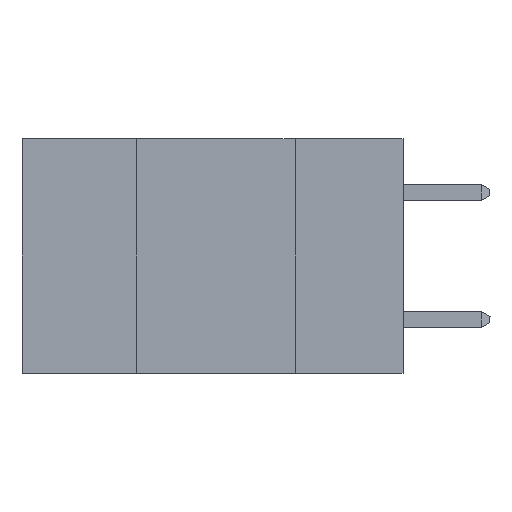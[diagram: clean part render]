
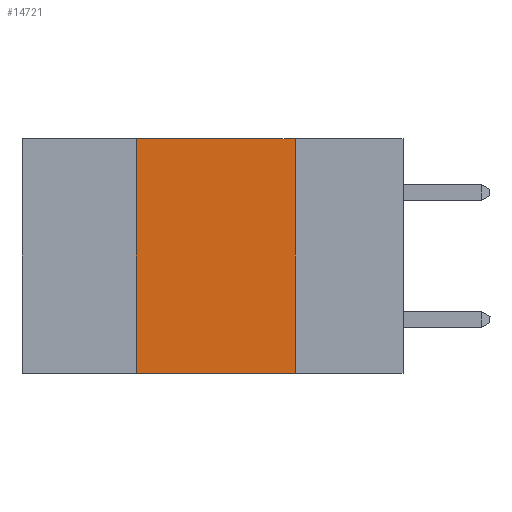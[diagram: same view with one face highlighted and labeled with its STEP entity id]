
A CAD part, left-side view. The second image highlights one B-rep face of the part: STEP entity #14721.
In plain terms, the highlighted planar face has unit normal (-1, 0, 0).
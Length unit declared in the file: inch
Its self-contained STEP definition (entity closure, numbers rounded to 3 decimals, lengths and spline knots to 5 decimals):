
#1542 = CARTESIAN_POINT ( 'NONE',  ( 0., 0.42, -0.37 ) ) ;
#1894 = LINE ( 'NONE', #10922, #10186 ) ;
#2434 = VERTEX_POINT ( 'NONE', #1542 ) ;
#3672 = DIRECTION ( 'NONE',  ( 0., -1., 0. ) ) ;
#5262 = ORIENTED_EDGE ( 'NONE', *, *, #19275, .T. ) ;
#6723 = VECTOR ( 'NONE', #13773, 39.37008 ) ;
#6943 = DIRECTION ( 'NONE',  ( 0., 0., 1. ) ) ;
#7241 = PLANE ( 'NONE',  #7673 ) ;
#7673 = AXIS2_PLACEMENT_3D ( 'NONE', #22280, #24285, #9198 ) ;
#8870 = VERTEX_POINT ( 'NONE', #21153 ) ;
#9198 = DIRECTION ( 'NONE',  ( 0., 0., -1. ) ) ;
#9713 = VECTOR ( 'NONE', #6943, 39.37008 ) ;
#10084 = VERTEX_POINT ( 'NONE', #17168 ) ;
#10186 = VECTOR ( 'NONE', #10846, 39.37008 ) ;
#10846 = DIRECTION ( 'NONE',  ( 0., -1., 0. ) ) ;
#10922 = CARTESIAN_POINT ( 'NONE',  ( 0., 0.6, -0.37 ) ) ;
#10974 = CARTESIAN_POINT ( 'NONE',  ( 0., 0.42, 0. ) ) ;
#11376 = CARTESIAN_POINT ( 'NONE',  ( 0., 0.17, 0. ) ) ;
#11456 = EDGE_CURVE ( 'NONE', #20526, #8870, #23297, .T. ) ;
#12977 = EDGE_LOOP ( 'NONE', ( #20979, #23933, #21020, #5262 ) ) ;
#13280 = CARTESIAN_POINT ( 'NONE',  ( 0., 0.6, 0. ) ) ;
#13773 = DIRECTION ( 'NONE',  ( 0., 0., -1. ) ) ;
#14094 = CARTESIAN_POINT ( 'NONE',  ( 0., 0.17, 0. ) ) ;
#14721 = ADVANCED_FACE ( 'NONE', ( #17850 ), #7241, .F. ) ;
#14800 = EDGE_CURVE ( 'NONE', #10084, #20526, #14871, .T. ) ;
#14871 = LINE ( 'NONE', #13280, #16642 ) ;
#16642 = VECTOR ( 'NONE', #3672, 39.37008 ) ;
#16869 = EDGE_CURVE ( 'NONE', #2434, #10084, #18344, .T. ) ;
#17168 = CARTESIAN_POINT ( 'NONE',  ( 0., 0.42, 0. ) ) ;
#17850 = FACE_OUTER_BOUND ( 'NONE', #12977, .T. ) ;
#18344 = LINE ( 'NONE', #10974, #9713 ) ;
#19275 = EDGE_CURVE ( 'NONE', #2434, #8870, #1894, .T. ) ;
#20526 = VERTEX_POINT ( 'NONE', #11376 ) ;
#20979 = ORIENTED_EDGE ( 'NONE', *, *, #11456, .F. ) ;
#21020 = ORIENTED_EDGE ( 'NONE', *, *, #16869, .F. ) ;
#21153 = CARTESIAN_POINT ( 'NONE',  ( 0., 0.17, -0.37 ) ) ;
#22280 = CARTESIAN_POINT ( 'NONE',  ( 0., 0.6, 0. ) ) ;
#23297 = LINE ( 'NONE', #14094, #6723 ) ;
#23933 = ORIENTED_EDGE ( 'NONE', *, *, #14800, .F. ) ;
#24285 = DIRECTION ( 'NONE',  ( 1., 0., 0. ) ) ;
